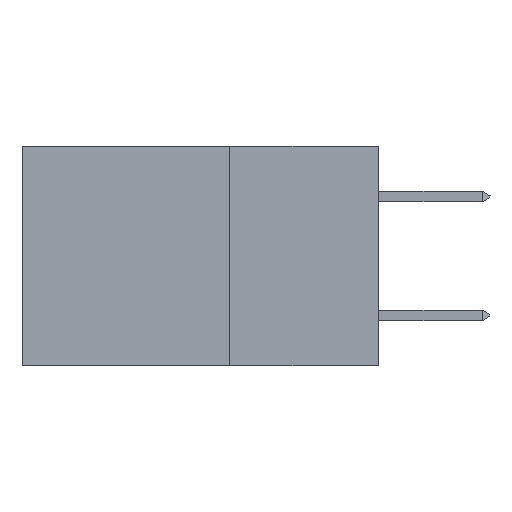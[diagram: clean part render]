
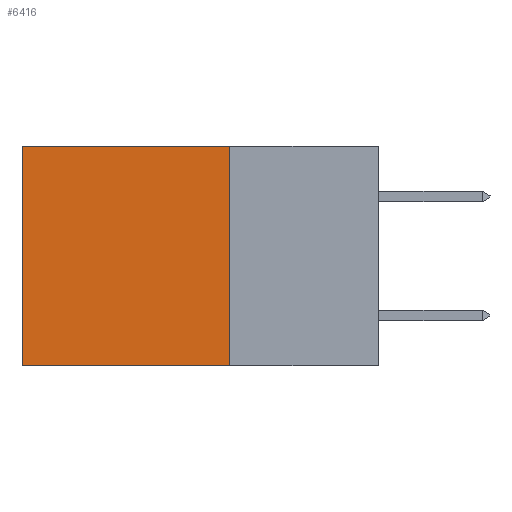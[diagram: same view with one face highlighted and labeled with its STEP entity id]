
A CAD part, left-side view. The second image highlights one B-rep face of the part: STEP entity #6416.
In plain terms, the highlighted planar face has unit normal (-1, 0, 0).
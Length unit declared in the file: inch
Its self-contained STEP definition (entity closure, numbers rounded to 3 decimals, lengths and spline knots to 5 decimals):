
#30 = EDGE_CURVE ( 'NONE', #12316, #18679, #19701, .T. ) ;
#185 = CARTESIAN_POINT ( 'NONE',  ( 0.2615, 0.6, -0.37 ) ) ;
#624 = DIRECTION ( 'NONE',  ( 0., 1., 0. ) ) ;
#1137 = CARTESIAN_POINT ( 'NONE',  ( 0.2615, 0.25, 0. ) ) ;
#1572 = VECTOR ( 'NONE', #15517, 39.37008 ) ;
#1651 = ORIENTED_EDGE ( 'NONE', *, *, #10494, .T. ) ;
#1833 = VECTOR ( 'NONE', #624, 39.37008 ) ;
#2073 = AXIS2_PLACEMENT_3D ( 'NONE', #24171, #3062, #10458 ) ;
#3034 = EDGE_LOOP ( 'NONE', ( #1651, #19781, #12330, #11670 ) ) ;
#3062 = DIRECTION ( 'NONE',  ( 1., 0., 0. ) ) ;
#4973 = LINE ( 'NONE', #1137, #1833 ) ;
#5517 = CARTESIAN_POINT ( 'NONE',  ( 0.2615, 0.25, -0.37 ) ) ;
#6416 = ADVANCED_FACE ( 'NONE', ( #17780 ), #10079, .F. ) ;
#7493 = EDGE_CURVE ( 'NONE', #23960, #12316, #22927, .T. ) ;
#7585 = LINE ( 'NONE', #21278, #9478 ) ;
#9478 = VECTOR ( 'NONE', #15545, 39.37008 ) ;
#9981 = CARTESIAN_POINT ( 'NONE',  ( 0.2615, 0.25, -0.37 ) ) ;
#10079 = PLANE ( 'NONE',  #2073 ) ;
#10458 = DIRECTION ( 'NONE',  ( 0., 0., -1. ) ) ;
#10494 = EDGE_CURVE ( 'NONE', #20747, #18679, #7585, .T. ) ;
#11670 = ORIENTED_EDGE ( 'NONE', *, *, #24646, .T. ) ;
#11864 = VECTOR ( 'NONE', #23299, 39.37008 ) ;
#11965 = CARTESIAN_POINT ( 'NONE',  ( 0.2615, 0.25, -0.37 ) ) ;
#12316 = VERTEX_POINT ( 'NONE', #9981 ) ;
#12330 = ORIENTED_EDGE ( 'NONE', *, *, #7493, .F. ) ;
#12421 = CARTESIAN_POINT ( 'NONE',  ( 0.2615, 0.6, 0. ) ) ;
#13891 = CARTESIAN_POINT ( 'NONE',  ( 0.2615, 0.25, 0. ) ) ;
#15517 = DIRECTION ( 'NONE',  ( 0., 1., 0. ) ) ;
#15545 = DIRECTION ( 'NONE',  ( 0., 0., -1. ) ) ;
#17780 = FACE_OUTER_BOUND ( 'NONE', #3034, .T. ) ;
#18679 = VERTEX_POINT ( 'NONE', #185 ) ;
#19701 = LINE ( 'NONE', #11965, #1572 ) ;
#19781 = ORIENTED_EDGE ( 'NONE', *, *, #30, .F. ) ;
#20747 = VERTEX_POINT ( 'NONE', #12421 ) ;
#21278 = CARTESIAN_POINT ( 'NONE',  ( 0.2615, 0.6, -0.37 ) ) ;
#22927 = LINE ( 'NONE', #5517, #11864 ) ;
#23299 = DIRECTION ( 'NONE',  ( 0., 0., -1. ) ) ;
#23960 = VERTEX_POINT ( 'NONE', #13891 ) ;
#24171 = CARTESIAN_POINT ( 'NONE',  ( 0.2615, 0.25, -0.37 ) ) ;
#24646 = EDGE_CURVE ( 'NONE', #23960, #20747, #4973, .T. ) ;
